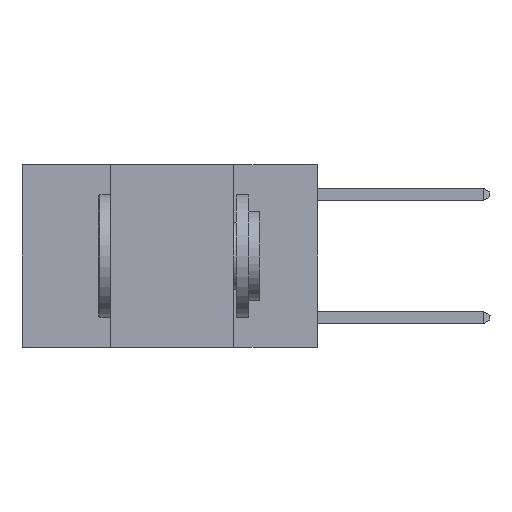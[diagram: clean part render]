
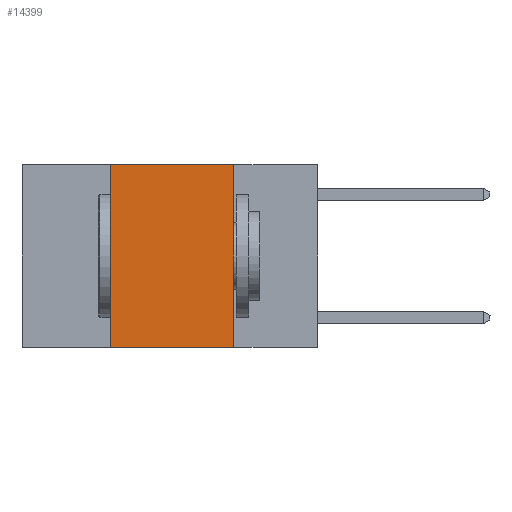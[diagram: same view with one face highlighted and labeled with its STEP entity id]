
A CAD part, left-side view. The second image highlights one B-rep face of the part: STEP entity #14399.
In plain terms, the highlighted planar face has unit normal (-1, 0, 0).
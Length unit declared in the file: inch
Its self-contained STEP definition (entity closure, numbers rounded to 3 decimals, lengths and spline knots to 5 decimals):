
#23 = DIRECTION ( 'NONE',  ( 0., -1., 0. ) ) ;
#461 = VERTEX_POINT ( 'NONE', #7588 ) ;
#682 = CARTESIAN_POINT ( 'NONE',  ( 0., 0.6, 0. ) ) ;
#688 = EDGE_CURVE ( 'NONE', #13312, #461, #3602, .T. ) ;
#1942 = ORIENTED_EDGE ( 'NONE', *, *, #10624, .F. ) ;
#2484 = AXIS2_PLACEMENT_3D ( 'NONE', #2748, #9828, #2807 ) ;
#2748 = CARTESIAN_POINT ( 'NONE',  ( 0., 0.6, 0. ) ) ;
#2807 = DIRECTION ( 'NONE',  ( 0., 0., -1. ) ) ;
#2815 = DIRECTION ( 'NONE',  ( 0., 0., 1. ) ) ;
#3602 = LINE ( 'NONE', #4434, #9782 ) ;
#4427 = LINE ( 'NONE', #10761, #7833 ) ;
#4434 = CARTESIAN_POINT ( 'NONE',  ( 0., 0.42, 0. ) ) ;
#4841 = ORIENTED_EDGE ( 'NONE', *, *, #688, .F. ) ;
#5313 = CARTESIAN_POINT ( 'NONE',  ( 0., 0.17, -0.37 ) ) ;
#6213 = DIRECTION ( 'NONE',  ( 0., 0., -1. ) ) ;
#7588 = CARTESIAN_POINT ( 'NONE',  ( 0., 0.42, 0. ) ) ;
#7833 = VECTOR ( 'NONE', #23, 39.37008 ) ;
#8489 = VECTOR ( 'NONE', #6213, 39.37008 ) ;
#8494 = EDGE_CURVE ( 'NONE', #13312, #14149, #4427, .T. ) ;
#8654 = PLANE ( 'NONE',  #2484 ) ;
#8941 = EDGE_CURVE ( 'NONE', #461, #11230, #14735, .T. ) ;
#9424 = CARTESIAN_POINT ( 'NONE',  ( 0., 0.17, 0. ) ) ;
#9728 = CARTESIAN_POINT ( 'NONE',  ( 0., 0.42, -0.37 ) ) ;
#9782 = VECTOR ( 'NONE', #2815, 39.37008 ) ;
#9828 = DIRECTION ( 'NONE',  ( 1., 0., 0. ) ) ;
#10376 = ORIENTED_EDGE ( 'NONE', *, *, #8941, .F. ) ;
#10624 = EDGE_CURVE ( 'NONE', #11230, #14149, #14700, .T. ) ;
#10761 = CARTESIAN_POINT ( 'NONE',  ( 0., 0.6, -0.37 ) ) ;
#11230 = VERTEX_POINT ( 'NONE', #9424 ) ;
#11425 = DIRECTION ( 'NONE',  ( 0., -1., 0. ) ) ;
#11689 = VECTOR ( 'NONE', #11425, 39.37008 ) ;
#11725 = FACE_OUTER_BOUND ( 'NONE', #11833, .T. ) ;
#11833 = EDGE_LOOP ( 'NONE', ( #1942, #10376, #4841, #14539 ) ) ;
#12053 = CARTESIAN_POINT ( 'NONE',  ( 0., 0.17, 0. ) ) ;
#13312 = VERTEX_POINT ( 'NONE', #9728 ) ;
#14149 = VERTEX_POINT ( 'NONE', #5313 ) ;
#14399 = ADVANCED_FACE ( 'NONE', ( #11725 ), #8654, .F. ) ;
#14539 = ORIENTED_EDGE ( 'NONE', *, *, #8494, .T. ) ;
#14700 = LINE ( 'NONE', #12053, #8489 ) ;
#14735 = LINE ( 'NONE', #682, #11689 ) ;
